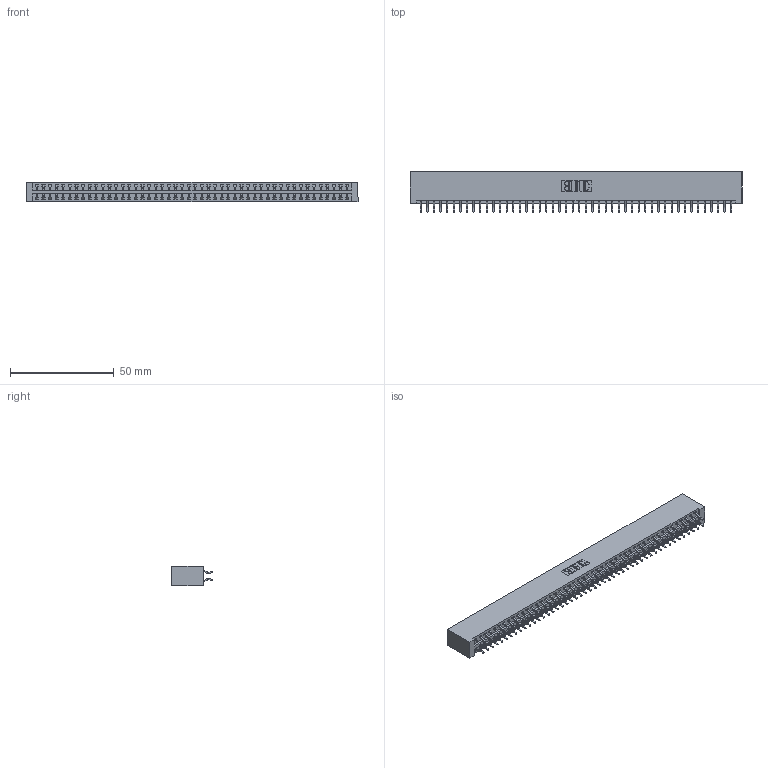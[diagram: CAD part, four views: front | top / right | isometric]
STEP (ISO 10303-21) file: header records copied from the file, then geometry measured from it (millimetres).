
FILE_DESCRIPTION (( 'STEP AP203' ), '1' );
FILE_NAME ('346-096-556-201.STEP', '2022-05-26T16:49:08', ( '' ), ( '' ), 'SwSTEP 2.0', 'SolidWorks 2020', '' );
FILE_SCHEMA (( 'CONFIG_CONTROL_DESIGN' ));
Length unit declared in the file: inch
Products named in the file (3): 346-096-556-201; 345-292-001_556 Tail; 346 Part_No Mounting Lugs
Assembly tree (97 placements, depth 2):
  346-096-556-201
    346 Part_No Mounting Lugs
    345-292-001_556 Tail  x96
Bounding box: 159.64 x 19.57 x 9.4 mm (x, y, z)
Volume: 16182.9 mm3; surface area: 22412.8 mm2
Topology: 97 solids, 97 shells, 5682 faces, 16913 edges, 11146 vertices
Faces by surface type: plane 3816, cylinder 1866
Entity records: 30461 total; most frequent: CARTESIAN_POINT 5024, ORIENTED_EDGE 4946, DIRECTION 4461, EDGE_CURVE 2473, LINE 2149, VECTOR 2149, VERTEX_POINT 1646, AXIS2_PLACEMENT_3D 1156
